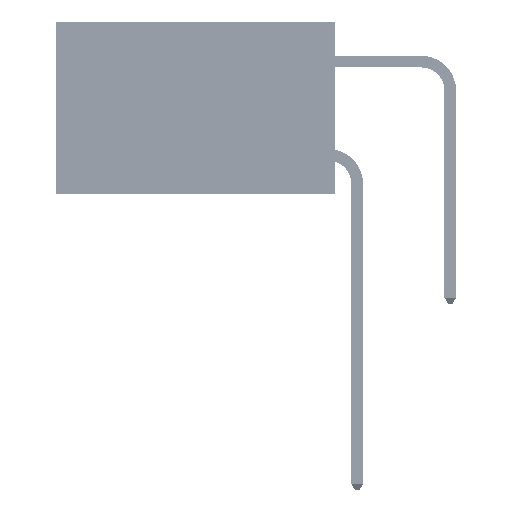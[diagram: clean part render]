
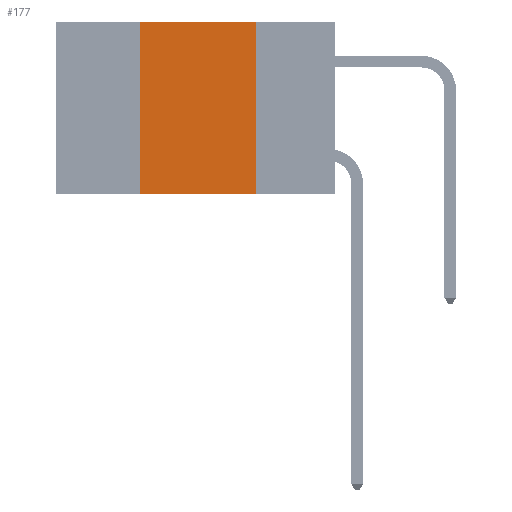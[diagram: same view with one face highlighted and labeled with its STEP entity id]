
A CAD part, left-side view. The second image highlights one B-rep face of the part: STEP entity #177.
In plain terms, the highlighted planar face has unit normal (-1, 0, 0).
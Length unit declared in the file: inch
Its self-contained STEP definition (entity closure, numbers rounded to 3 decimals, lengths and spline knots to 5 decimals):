
#177 = ADVANCED_FACE ( 'NONE', ( #33122 ), #32202, .F. ) ;
#4263 = VERTEX_POINT ( 'NONE', #19422 ) ;
#5122 = VERTEX_POINT ( 'NONE', #49264 ) ;
#7789 = DIRECTION ( 'NONE',  ( 0., -1., 0. ) ) ;
#8162 = LINE ( 'NONE', #38485, #33731 ) ;
#10537 = EDGE_CURVE ( 'NONE', #4263, #23093, #12347, .T. ) ;
#10992 = ORIENTED_EDGE ( 'NONE', *, *, #16952, .T. ) ;
#12033 = ORIENTED_EDGE ( 'NONE', *, *, #48177, .F. ) ;
#12347 = LINE ( 'NONE', #22573, #28156 ) ;
#12552 = VECTOR ( 'NONE', #46981, 39.37008 ) ;
#12972 = DIRECTION ( 'NONE',  ( 0., 0., -1. ) ) ;
#13132 = CARTESIAN_POINT ( 'NONE',  ( 0., 0.6, 0. ) ) ;
#15798 = CARTESIAN_POINT ( 'NONE',  ( 0., 0.17, 0. ) ) ;
#16307 = VECTOR ( 'NONE', #24356, 39.37008 ) ;
#16952 = EDGE_CURVE ( 'NONE', #31267, #5122, #20569, .T. ) ;
#18329 = AXIS2_PLACEMENT_3D ( 'NONE', #13132, #20278, #12972 ) ;
#19422 = CARTESIAN_POINT ( 'NONE',  ( 0., 0.42, 0. ) ) ;
#20278 = DIRECTION ( 'NONE',  ( 1., 0., 0. ) ) ;
#20569 = LINE ( 'NONE', #40495, #16307 ) ;
#22573 = CARTESIAN_POINT ( 'NONE',  ( 0., 0.6, 0. ) ) ;
#23093 = VERTEX_POINT ( 'NONE', #34580 ) ;
#24356 = DIRECTION ( 'NONE',  ( 0., -1., 0. ) ) ;
#28156 = VECTOR ( 'NONE', #7789, 39.37008 ) ;
#31267 = VERTEX_POINT ( 'NONE', #38840 ) ;
#32202 = PLANE ( 'NONE',  #18329 ) ;
#33122 = FACE_OUTER_BOUND ( 'NONE', #49817, .T. ) ;
#33731 = VECTOR ( 'NONE', #42587, 39.37008 ) ;
#34580 = CARTESIAN_POINT ( 'NONE',  ( 0., 0.17, 0. ) ) ;
#38134 = EDGE_CURVE ( 'NONE', #31267, #4263, #8162, .T. ) ;
#38485 = CARTESIAN_POINT ( 'NONE',  ( 0., 0.42, 0. ) ) ;
#38840 = CARTESIAN_POINT ( 'NONE',  ( 0., 0.42, -0.37 ) ) ;
#40495 = CARTESIAN_POINT ( 'NONE',  ( 0., 0.6, -0.37 ) ) ;
#42587 = DIRECTION ( 'NONE',  ( 0., 0., 1. ) ) ;
#46981 = DIRECTION ( 'NONE',  ( 0., 0., -1. ) ) ;
#47812 = LINE ( 'NONE', #15798, #12552 ) ;
#48177 = EDGE_CURVE ( 'NONE', #23093, #5122, #47812, .T. ) ;
#49105 = ORIENTED_EDGE ( 'NONE', *, *, #38134, .F. ) ;
#49264 = CARTESIAN_POINT ( 'NONE',  ( 0., 0.17, -0.37 ) ) ;
#49817 = EDGE_LOOP ( 'NONE', ( #12033, #50224, #49105, #10992 ) ) ;
#50224 = ORIENTED_EDGE ( 'NONE', *, *, #10537, .F. ) ;
